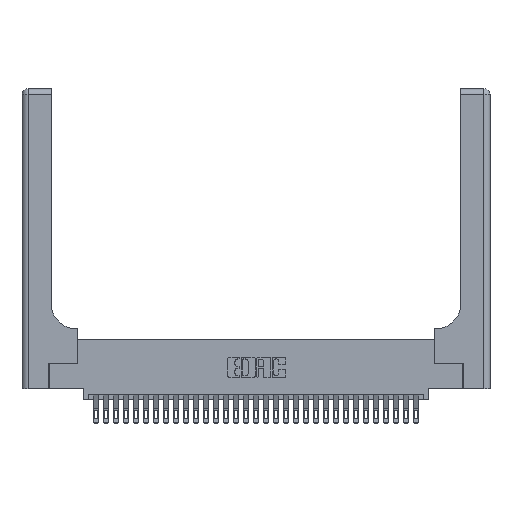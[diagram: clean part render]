
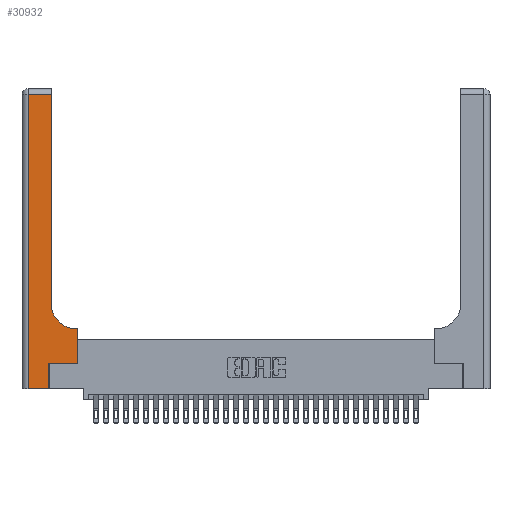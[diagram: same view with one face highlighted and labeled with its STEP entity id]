
A CAD part, top view. The second image highlights one B-rep face of the part: STEP entity #30932.
In plain terms, the highlighted planar face has unit normal (0, 0, 1).
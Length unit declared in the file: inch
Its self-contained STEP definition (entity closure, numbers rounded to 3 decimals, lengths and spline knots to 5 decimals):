
#178 = VECTOR ( 'NONE', #15911, 39.37008 ) ;
#359 = ORIENTED_EDGE ( 'NONE', *, *, #29101, .T. ) ;
#491 = CARTESIAN_POINT ( 'NONE',  ( 0., 2.94, 0.37 ) ) ;
#989 = CARTESIAN_POINT ( 'NONE',  ( 0.269, 0., 0.37 ) ) ;
#1947 = ORIENTED_EDGE ( 'NONE', *, *, #8047, .T. ) ;
#1977 = DIRECTION ( 'NONE',  ( 1., 0., 0. ) ) ;
#2136 = VECTOR ( 'NONE', #25230, 39.37008 ) ;
#2697 = VERTEX_POINT ( 'NONE', #8814 ) ;
#2789 = VECTOR ( 'NONE', #20867, 39.37008 ) ;
#3143 = ORIENTED_EDGE ( 'NONE', *, *, #29923, .T. ) ;
#3671 = CARTESIAN_POINT ( 'NONE',  ( 0.269, 0.25, 0.37 ) ) ;
#5069 = CARTESIAN_POINT ( 'NONE',  ( 0., 3., 0.37 ) ) ;
#5370 = EDGE_CURVE ( 'NONE', #31535, #2697, #16604, .T. ) ;
#5662 = DIRECTION ( 'NONE',  ( -1., 0., 0. ) ) ;
#6129 = DIRECTION ( 'NONE',  ( -1., 0., 0. ) ) ;
#7364 = VECTOR ( 'NONE', #28653, 39.37008 ) ;
#7747 = CARTESIAN_POINT ( 'NONE',  ( 0.2915, 3., 0.37 ) ) ;
#8047 = EDGE_CURVE ( 'NONE', #20991, #32182, #8948, .T. ) ;
#8376 = VERTEX_POINT ( 'NONE', #989 ) ;
#8461 = CARTESIAN_POINT ( 'NONE',  ( 0.5585, 0.25, 0.37 ) ) ;
#8547 = VERTEX_POINT ( 'NONE', #11842 ) ;
#8763 = VECTOR ( 'NONE', #5662, 39.37008 ) ;
#8814 = CARTESIAN_POINT ( 'NONE',  ( 0.2915, 0.85, 0.37 ) ) ;
#8948 = LINE ( 'NONE', #20153, #2136 ) ;
#11842 = CARTESIAN_POINT ( 'NONE',  ( 0.5585, 0.25, 0.37 ) ) ;
#12769 = PLANE ( 'NONE',  #22747 ) ;
#12876 = DIRECTION ( 'NONE',  ( -1., 0., 0. ) ) ;
#13394 = CARTESIAN_POINT ( 'NONE',  ( 0.269, 0., 0.37 ) ) ;
#13960 = VERTEX_POINT ( 'NONE', #3671 ) ;
#14892 = DIRECTION ( 'NONE',  ( 0., 0., -1. ) ) ;
#14951 = VECTOR ( 'NONE', #1977, 39.37008 ) ;
#15271 = CARTESIAN_POINT ( 'NONE',  ( 0.5415, 0.85, 0.37 ) ) ;
#15911 = DIRECTION ( 'NONE',  ( 0., 1., 0. ) ) ;
#16220 = CARTESIAN_POINT ( 'NONE',  ( 0.2915, 0.6, 0.37 ) ) ;
#16306 = ORIENTED_EDGE ( 'NONE', *, *, #20745, .T. ) ;
#16604 = CIRCLE ( 'NONE', #30202, 0.25 ) ;
#17146 = LINE ( 'NONE', #23296, #2789 ) ;
#17250 = CARTESIAN_POINT ( 'NONE',  ( 0.269, 0.25, 0.37 ) ) ;
#17276 = EDGE_CURVE ( 'NONE', #28506, #20991, #23031, .T. ) ;
#17786 = DIRECTION ( 'NONE',  ( 1., 0., 0. ) ) ;
#18113 = CARTESIAN_POINT ( 'NONE',  ( 0.06, 2.94, 0.37 ) ) ;
#18168 = VECTOR ( 'NONE', #27929, 39.37008 ) ;
#18282 = ORIENTED_EDGE ( 'NONE', *, *, #32305, .T. ) ;
#18651 = EDGE_LOOP ( 'NONE', ( #359, #20654, #1947, #23026, #21837, #16306, #18282, #3143, #21023 ) ) ;
#20153 = CARTESIAN_POINT ( 'NONE',  ( 0.06, 3., 0.37 ) ) ;
#20470 = LINE ( 'NONE', #13394, #178 ) ;
#20654 = ORIENTED_EDGE ( 'NONE', *, *, #17276, .T. ) ;
#20745 = EDGE_CURVE ( 'NONE', #13960, #8547, #20819, .T. ) ;
#20815 = LINE ( 'NONE', #8461, #7364 ) ;
#20819 = LINE ( 'NONE', #17250, #14951 ) ;
#20867 = DIRECTION ( 'NONE',  ( 1., 0., 0. ) ) ;
#20991 = VERTEX_POINT ( 'NONE', #18113 ) ;
#21023 = ORIENTED_EDGE ( 'NONE', *, *, #5370, .T. ) ;
#21837 = ORIENTED_EDGE ( 'NONE', *, *, #31626, .T. ) ;
#22573 = EDGE_CURVE ( 'NONE', #32182, #8376, #17146, .T. ) ;
#22747 = AXIS2_PLACEMENT_3D ( 'NONE', #5069, #27935, #12876 ) ;
#23026 = ORIENTED_EDGE ( 'NONE', *, *, #22573, .T. ) ;
#23031 = LINE ( 'NONE', #491, #8763 ) ;
#23296 = CARTESIAN_POINT ( 'NONE',  ( 0., 0., 0.37 ) ) ;
#23343 = VECTOR ( 'NONE', #6129, 39.37008 ) ;
#25230 = DIRECTION ( 'NONE',  ( 0., -1., 0. ) ) ;
#26706 = VERTEX_POINT ( 'NONE', #30674 ) ;
#27599 = FACE_OUTER_BOUND ( 'NONE', #18651, .T. ) ;
#27929 = DIRECTION ( 'NONE',  ( 0., 1., 0. ) ) ;
#27935 = DIRECTION ( 'NONE',  ( 0., 0., -1. ) ) ;
#28116 = CARTESIAN_POINT ( 'NONE',  ( 0.5415, 0.6, 0.37 ) ) ;
#28506 = VERTEX_POINT ( 'NONE', #32776 ) ;
#28653 = DIRECTION ( 'NONE',  ( 0., 1., 0. ) ) ;
#29101 = EDGE_CURVE ( 'NONE', #2697, #28506, #31487, .T. ) ;
#29923 = EDGE_CURVE ( 'NONE', #26706, #31535, #30001, .T. ) ;
#30001 = LINE ( 'NONE', #16220, #23343 ) ;
#30202 = AXIS2_PLACEMENT_3D ( 'NONE', #15271, #14892, #17786 ) ;
#30621 = CARTESIAN_POINT ( 'NONE',  ( 0.06, 0., 0.37 ) ) ;
#30674 = CARTESIAN_POINT ( 'NONE',  ( 0.5585, 0.6, 0.37 ) ) ;
#30932 = ADVANCED_FACE ( 'NONE', ( #27599 ), #12769, .F. ) ;
#31487 = LINE ( 'NONE', #7747, #18168 ) ;
#31535 = VERTEX_POINT ( 'NONE', #28116 ) ;
#31626 = EDGE_CURVE ( 'NONE', #8376, #13960, #20470, .T. ) ;
#32182 = VERTEX_POINT ( 'NONE', #30621 ) ;
#32305 = EDGE_CURVE ( 'NONE', #8547, #26706, #20815, .T. ) ;
#32776 = CARTESIAN_POINT ( 'NONE',  ( 0.2915, 2.94, 0.37 ) ) ;
